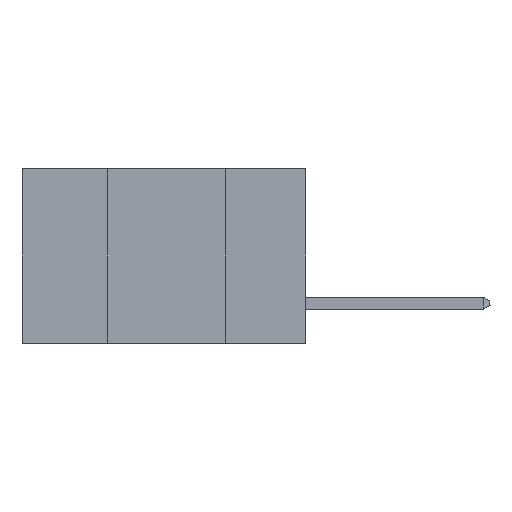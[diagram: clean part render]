
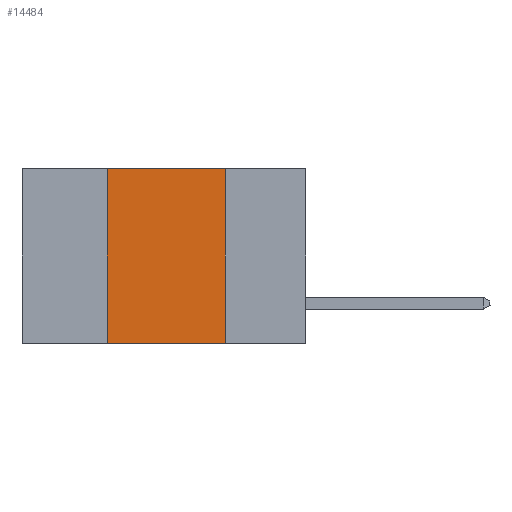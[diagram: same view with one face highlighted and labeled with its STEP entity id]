
A CAD part, left-side view. The second image highlights one B-rep face of the part: STEP entity #14484.
In plain terms, the highlighted planar face has unit normal (-1, 0, 0).
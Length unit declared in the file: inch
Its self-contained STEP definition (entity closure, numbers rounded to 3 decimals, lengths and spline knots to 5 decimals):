
#1534 = CARTESIAN_POINT ( 'NONE',  ( 0., 0.6, 0. ) ) ;
#2017 = CARTESIAN_POINT ( 'NONE',  ( 0., 0.17, 0. ) ) ;
#2592 = EDGE_CURVE ( 'NONE', #17857, #28908, #21819, .T. ) ;
#4546 = VECTOR ( 'NONE', #22491, 39.37008 ) ;
#4709 = ORIENTED_EDGE ( 'NONE', *, *, #2592, .T. ) ;
#5266 = EDGE_LOOP ( 'NONE', ( #21671, #28918, #18550, #4709 ) ) ;
#6208 = CARTESIAN_POINT ( 'NONE',  ( 0., 0.42, 0. ) ) ;
#7457 = EDGE_CURVE ( 'NONE', #17857, #9340, #12940, .T. ) ;
#7725 = CARTESIAN_POINT ( 'NONE',  ( 0., 0.17, 0. ) ) ;
#7819 = LINE ( 'NONE', #2017, #10344 ) ;
#7894 = DIRECTION ( 'NONE',  ( 0., -1., 0. ) ) ;
#8211 = EDGE_CURVE ( 'NONE', #11937, #28908, #7819, .T. ) ;
#9340 = VERTEX_POINT ( 'NONE', #11417 ) ;
#10344 = VECTOR ( 'NONE', #20709, 39.37008 ) ;
#11417 = CARTESIAN_POINT ( 'NONE',  ( 0., 0.42, 0. ) ) ;
#11937 = VERTEX_POINT ( 'NONE', #7725 ) ;
#12600 = LINE ( 'NONE', #19507, #24209 ) ;
#12940 = LINE ( 'NONE', #6208, #4546 ) ;
#14484 = ADVANCED_FACE ( 'NONE', ( #15158 ), #15480, .F. ) ;
#14720 = CARTESIAN_POINT ( 'NONE',  ( 0., 0.6, -0.37 ) ) ;
#15158 = FACE_OUTER_BOUND ( 'NONE', #5266, .T. ) ;
#15480 = PLANE ( 'NONE',  #21824 ) ;
#17857 = VERTEX_POINT ( 'NONE', #17963 ) ;
#17963 = CARTESIAN_POINT ( 'NONE',  ( 0., 0.42, -0.37 ) ) ;
#18550 = ORIENTED_EDGE ( 'NONE', *, *, #7457, .F. ) ;
#19507 = CARTESIAN_POINT ( 'NONE',  ( 0., 0.6, 0. ) ) ;
#20028 = VECTOR ( 'NONE', #21584, 39.37008 ) ;
#20709 = DIRECTION ( 'NONE',  ( 0., 0., -1. ) ) ;
#21507 = CARTESIAN_POINT ( 'NONE',  ( 0., 0.17, -0.37 ) ) ;
#21584 = DIRECTION ( 'NONE',  ( 0., -1., 0. ) ) ;
#21671 = ORIENTED_EDGE ( 'NONE', *, *, #8211, .F. ) ;
#21819 = LINE ( 'NONE', #14720, #20028 ) ;
#21824 = AXIS2_PLACEMENT_3D ( 'NONE', #1534, #27129, #22253 ) ;
#22253 = DIRECTION ( 'NONE',  ( 0., 0., -1. ) ) ;
#22491 = DIRECTION ( 'NONE',  ( 0., 0., 1. ) ) ;
#24209 = VECTOR ( 'NONE', #7894, 39.37008 ) ;
#27106 = EDGE_CURVE ( 'NONE', #9340, #11937, #12600, .T. ) ;
#27129 = DIRECTION ( 'NONE',  ( 1., 0., 0. ) ) ;
#28908 = VERTEX_POINT ( 'NONE', #21507 ) ;
#28918 = ORIENTED_EDGE ( 'NONE', *, *, #27106, .F. ) ;
